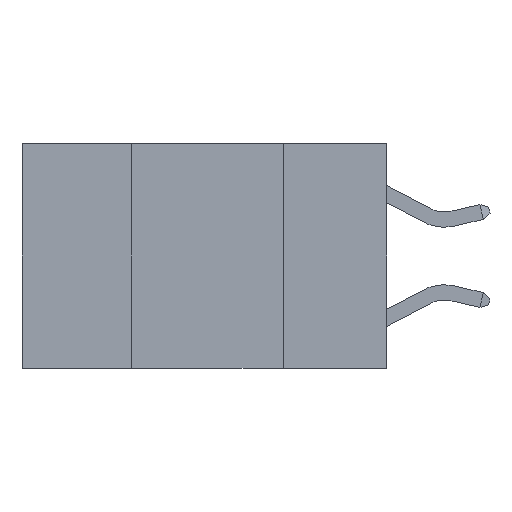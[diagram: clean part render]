
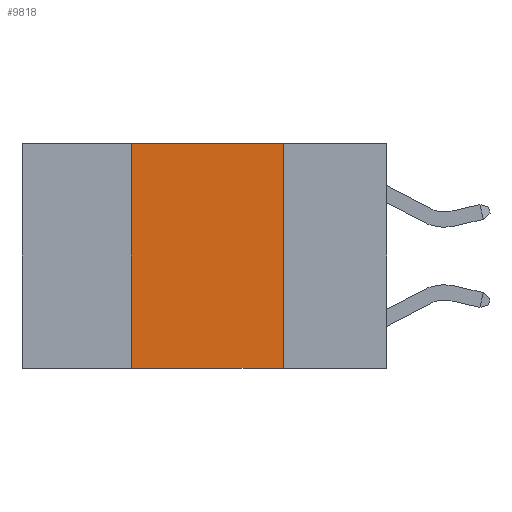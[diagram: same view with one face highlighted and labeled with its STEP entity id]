
A CAD part, left-side view. The second image highlights one B-rep face of the part: STEP entity #9818.
In plain terms, the highlighted planar face has unit normal (-1, 0, 0).
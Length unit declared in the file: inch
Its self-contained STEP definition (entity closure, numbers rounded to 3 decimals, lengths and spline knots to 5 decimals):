
#28 = DIRECTION ( 'NONE',  ( 0., -1., 0. ) ) ;
#152 = CARTESIAN_POINT ( 'NONE',  ( 0., 0.17, 0. ) ) ;
#285 = VECTOR ( 'NONE', #8136, 39.37008 ) ;
#294 = ORIENTED_EDGE ( 'NONE', *, *, #9461, .F. ) ;
#362 = DIRECTION ( 'NONE',  ( 0., 0., 1. ) ) ;
#739 = ORIENTED_EDGE ( 'NONE', *, *, #1304, .F. ) ;
#777 = VERTEX_POINT ( 'NONE', #2569 ) ;
#1258 = FACE_OUTER_BOUND ( 'NONE', #10798, .T. ) ;
#1304 = EDGE_CURVE ( 'NONE', #777, #5736, #9235, .T. ) ;
#1411 = CARTESIAN_POINT ( 'NONE',  ( 0., 0.42, 0. ) ) ;
#2569 = CARTESIAN_POINT ( 'NONE',  ( 0., 0.17, 0. ) ) ;
#2955 = LINE ( 'NONE', #6905, #9269 ) ;
#3020 = CARTESIAN_POINT ( 'NONE',  ( 0., 0.42, 0. ) ) ;
#3427 = VECTOR ( 'NONE', #9774, 39.37008 ) ;
#3896 = ORIENTED_EDGE ( 'NONE', *, *, #5556, .T. ) ;
#4088 = AXIS2_PLACEMENT_3D ( 'NONE', #9215, #10002, #5159 ) ;
#4218 = CARTESIAN_POINT ( 'NONE',  ( 0., 0.42, -0.37 ) ) ;
#5159 = DIRECTION ( 'NONE',  ( 0., 0., -1. ) ) ;
#5556 = EDGE_CURVE ( 'NONE', #8463, #5736, #2955, .T. ) ;
#5736 = VERTEX_POINT ( 'NONE', #6375 ) ;
#6375 = CARTESIAN_POINT ( 'NONE',  ( 0., 0.17, -0.37 ) ) ;
#6553 = CARTESIAN_POINT ( 'NONE',  ( 0., 0.6, 0. ) ) ;
#6723 = LINE ( 'NONE', #6553, #3427 ) ;
#6905 = CARTESIAN_POINT ( 'NONE',  ( 0., 0.6, -0.37 ) ) ;
#7224 = LINE ( 'NONE', #3020, #9108 ) ;
#7722 = EDGE_CURVE ( 'NONE', #9515, #777, #6723, .T. ) ;
#8136 = DIRECTION ( 'NONE',  ( 0., 0., -1. ) ) ;
#8463 = VERTEX_POINT ( 'NONE', #4218 ) ;
#8832 = ORIENTED_EDGE ( 'NONE', *, *, #7722, .F. ) ;
#9108 = VECTOR ( 'NONE', #362, 39.37008 ) ;
#9215 = CARTESIAN_POINT ( 'NONE',  ( 0., 0.6, 0. ) ) ;
#9235 = LINE ( 'NONE', #152, #285 ) ;
#9269 = VECTOR ( 'NONE', #28, 39.37008 ) ;
#9461 = EDGE_CURVE ( 'NONE', #8463, #9515, #7224, .T. ) ;
#9515 = VERTEX_POINT ( 'NONE', #1411 ) ;
#9774 = DIRECTION ( 'NONE',  ( 0., -1., 0. ) ) ;
#9818 = ADVANCED_FACE ( 'NONE', ( #1258 ), #10783, .F. ) ;
#10002 = DIRECTION ( 'NONE',  ( 1., 0., 0. ) ) ;
#10783 = PLANE ( 'NONE',  #4088 ) ;
#10798 = EDGE_LOOP ( 'NONE', ( #739, #8832, #294, #3896 ) ) ;
